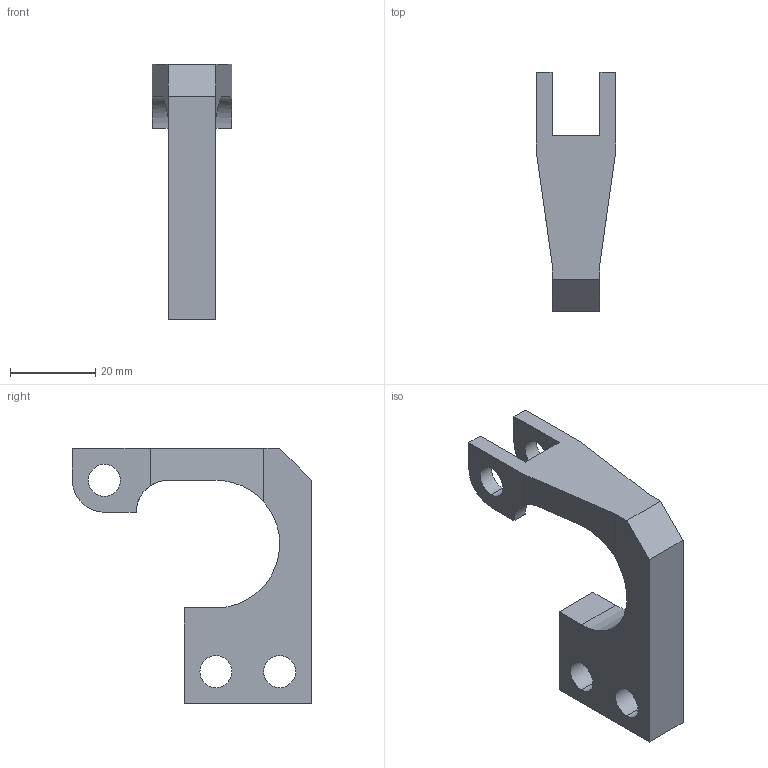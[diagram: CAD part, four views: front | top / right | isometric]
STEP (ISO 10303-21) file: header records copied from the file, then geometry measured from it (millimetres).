
FILE_DESCRIPTION (( 'STEP AP203' ), '1' );
FILE_NAME ('Trigger_Guard.STEP', '2013-09-22T12:17:59', ( '' ), ( '' ), 'SwSTEP 2.0', 'SolidWorks 2013', '' );
FILE_SCHEMA (( 'CONFIG_CONTROL_DESIGN' ));
Length unit declared in the file: millimetre
Products named in the file (1): Trigger_Guard
Bounding box: 18.75 x 56.25 x 60 mm (x, y, z)
Volume: 15687.5 mm3; surface area: 6999.8 mm2
Topology: 1 solids, 1 shells, 34 faces, 96 edges, 64 vertices
Faces by surface type: plane 20, cylinder 14
Entity records: 1201 total; most frequent: CARTESIAN_POINT 207, ORIENTED_EDGE 192, DIRECTION 190, EDGE_CURVE 96, VERTEX_POINT 64, VECTOR 64, LINE 64, AXIS2_PLACEMENT_3D 63
